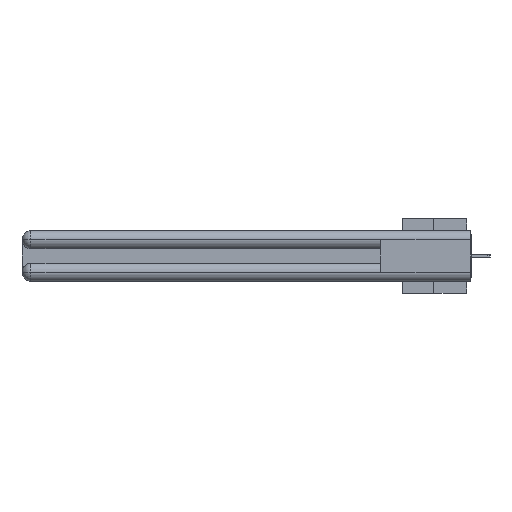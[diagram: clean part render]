
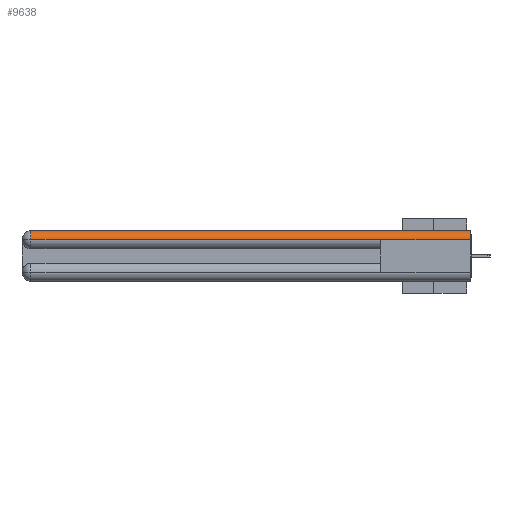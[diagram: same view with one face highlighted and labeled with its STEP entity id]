
A CAD part, left-side view. The second image highlights one B-rep face of the part: STEP entity #9638.
In plain terms, the highlighted cylindrical face has radius 1.562 mm (diameter 3.124 mm), a partial arc.
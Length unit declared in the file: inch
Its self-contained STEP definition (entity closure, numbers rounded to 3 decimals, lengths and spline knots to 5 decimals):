
#153 = DIRECTION ( 'NONE',  ( 0., -1., 0. ) ) ;
#659 = DIRECTION ( 'NONE',  ( 0., 0., 1. ) ) ;
#698 = CARTESIAN_POINT ( 'NONE',  ( 0., 0., -0.0615 ) ) ;
#1240 = CARTESIAN_POINT ( 'NONE',  ( 0., 2.94, -0.0615 ) ) ;
#2008 = EDGE_CURVE ( 'NONE', #33799, #7440, #19832, .T. ) ;
#3559 = EDGE_LOOP ( 'NONE', ( #7109, #14477, #30875, #25471, #33724 ) ) ;
#4316 = AXIS2_PLACEMENT_3D ( 'NONE', #26555, #26548, #26322 ) ;
#6974 = CARTESIAN_POINT ( 'NONE',  ( 0., 3., -0.0615 ) ) ;
#7055 = FACE_OUTER_BOUND ( 'NONE', #3559, .T. ) ;
#7109 = ORIENTED_EDGE ( 'NONE', *, *, #8234, .F. ) ;
#7440 = VERTEX_POINT ( 'NONE', #1240 ) ;
#8234 = EDGE_CURVE ( 'NONE', #33799, #14492, #30004, .T. ) ;
#9638 = ADVANCED_FACE ( 'NONE', ( #7055 ), #27478, .T. ) ;
#14477 = ORIENTED_EDGE ( 'NONE', *, *, #2008, .T. ) ;
#14492 = VERTEX_POINT ( 'NONE', #17660 ) ;
#15433 = VECTOR ( 'NONE', #20646, 39.37008 ) ;
#15719 = DIRECTION ( 'NONE',  ( 0., -1., 0. ) ) ;
#15963 = VECTOR ( 'NONE', #15719, 39.37008 ) ;
#16276 = CARTESIAN_POINT ( 'NONE',  ( 0.0615, 0., -0.0615 ) ) ;
#16776 = CARTESIAN_POINT ( 'NONE',  ( 0.0615, 0., -0.0615 ) ) ;
#17660 = CARTESIAN_POINT ( 'NONE',  ( 0.0615, 0., 0. ) ) ;
#17815 = EDGE_CURVE ( 'NONE', #23754, #29840, #29500, .T. ) ;
#18904 = DIRECTION ( 'NONE',  ( 1., 0., 0. ) ) ;
#19738 = EDGE_CURVE ( 'NONE', #14492, #23754, #30159, .T. ) ;
#19832 = CIRCLE ( 'NONE', #4316, 0.0615 ) ;
#20646 = DIRECTION ( 'NONE',  ( 0., 1., 0. ) ) ;
#22844 = CARTESIAN_POINT ( 'NONE',  ( 0., 0.6, -0.0615 ) ) ;
#23328 = CARTESIAN_POINT ( 'NONE',  ( 0.0615, 2.94, 0. ) ) ;
#23754 = VERTEX_POINT ( 'NONE', #698 ) ;
#25471 = ORIENTED_EDGE ( 'NONE', *, *, #17815, .F. ) ;
#26289 = CARTESIAN_POINT ( 'NONE',  ( 0.0615, 0., 0. ) ) ;
#26322 = DIRECTION ( 'NONE',  ( 0., 0., 1. ) ) ;
#26548 = DIRECTION ( 'NONE',  ( 0., -1., 0. ) ) ;
#26555 = CARTESIAN_POINT ( 'NONE',  ( 0.0615, 2.94, -0.0615 ) ) ;
#27478 = CYLINDRICAL_SURFACE ( 'NONE', #32116, 0.0615 ) ;
#28282 = DIRECTION ( 'NONE',  ( 0., -1., 0. ) ) ;
#28410 = LINE ( 'NONE', #6974, #32878 ) ;
#29500 = LINE ( 'NONE', #31142, #15433 ) ;
#29840 = VERTEX_POINT ( 'NONE', #22844 ) ;
#29874 = EDGE_CURVE ( 'NONE', #7440, #29840, #28410, .T. ) ;
#29952 = DIRECTION ( 'NONE',  ( 0., 1., 0. ) ) ;
#30004 = LINE ( 'NONE', #26289, #15963 ) ;
#30159 = CIRCLE ( 'NONE', #34371, 0.0615 ) ;
#30875 = ORIENTED_EDGE ( 'NONE', *, *, #29874, .T. ) ;
#31142 = CARTESIAN_POINT ( 'NONE',  ( 0., 3., -0.0615 ) ) ;
#32116 = AXIS2_PLACEMENT_3D ( 'NONE', #16776, #29952, #659 ) ;
#32878 = VECTOR ( 'NONE', #28282, 39.37008 ) ;
#33724 = ORIENTED_EDGE ( 'NONE', *, *, #19738, .F. ) ;
#33799 = VERTEX_POINT ( 'NONE', #23328 ) ;
#34371 = AXIS2_PLACEMENT_3D ( 'NONE', #16276, #153, #18904 ) ;
